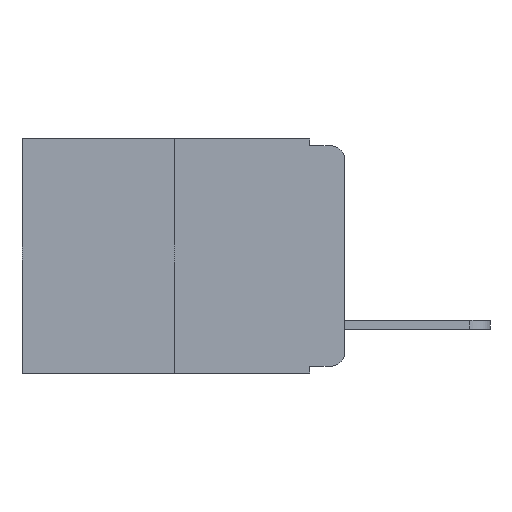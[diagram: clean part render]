
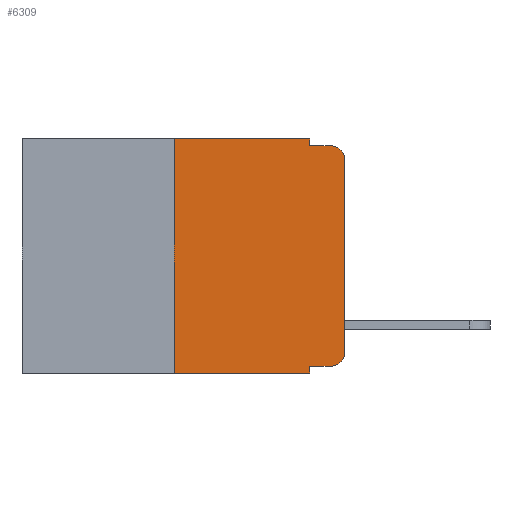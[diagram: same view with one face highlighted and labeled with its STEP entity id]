
A CAD part, left-side view. The second image highlights one B-rep face of the part: STEP entity #6309.
In plain terms, the highlighted planar face has unit normal (-1, 0, 0).
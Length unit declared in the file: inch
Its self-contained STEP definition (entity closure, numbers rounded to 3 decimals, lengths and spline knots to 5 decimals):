
#97 = EDGE_CURVE ( 'NONE', #1226, #12075, #10410, .T. ) ;
#173 = CARTESIAN_POINT ( 'NONE',  ( 0., 0.051, 0. ) ) ;
#277 = EDGE_CURVE ( 'NONE', #12075, #1730, #10878, .T. ) ;
#729 = VERTEX_POINT ( 'NONE', #4508 ) ;
#790 = VECTOR ( 'NONE', #1117, 39.37008 ) ;
#823 = ORIENTED_EDGE ( 'NONE', *, *, #1508, .T. ) ;
#833 = VERTEX_POINT ( 'NONE', #1944 ) ;
#1117 = DIRECTION ( 'NONE',  ( 0., 0., 1. ) ) ;
#1226 = VERTEX_POINT ( 'NONE', #11450 ) ;
#1508 = EDGE_CURVE ( 'NONE', #1730, #5618, #3869, .T. ) ;
#1667 = DIRECTION ( 'NONE',  ( 0., 0., -1. ) ) ;
#1677 = DIRECTION ( 'NONE',  ( -1., 0., 0. ) ) ;
#1699 = CARTESIAN_POINT ( 'NONE',  ( 0., 0.02, -0.313 ) ) ;
#1730 = VERTEX_POINT ( 'NONE', #4477 ) ;
#1927 = ORIENTED_EDGE ( 'NONE', *, *, #9989, .F. ) ;
#1944 = CARTESIAN_POINT ( 'NONE',  ( 0., 0.25, -0.343 ) ) ;
#1975 = VECTOR ( 'NONE', #6902, 39.37008 ) ;
#1986 = CARTESIAN_POINT ( 'NONE',  ( 0., 0., 0. ) ) ;
#2204 = AXIS2_PLACEMENT_3D ( 'NONE', #10571, #10408, #10288 ) ;
#2370 = CARTESIAN_POINT ( 'NONE',  ( 0., 0.25, 0. ) ) ;
#2376 = CARTESIAN_POINT ( 'NONE',  ( 0., 0.02, -0.333 ) ) ;
#2549 = LINE ( 'NONE', #5717, #13097 ) ;
#2639 = VERTEX_POINT ( 'NONE', #9221 ) ;
#2655 = ORIENTED_EDGE ( 'NONE', *, *, #7296, .F. ) ;
#3625 = LINE ( 'NONE', #7556, #9122 ) ;
#3672 = VECTOR ( 'NONE', #12641, 39.37008 ) ;
#3692 = VERTEX_POINT ( 'NONE', #173 ) ;
#3740 = ORIENTED_EDGE ( 'NONE', *, *, #12551, .T. ) ;
#3869 = LINE ( 'NONE', #1986, #790 ) ;
#3941 = CARTESIAN_POINT ( 'NONE',  ( 0., 0., -0.03 ) ) ;
#4017 = VERTEX_POINT ( 'NONE', #8702 ) ;
#4297 = DIRECTION ( 'NONE',  ( 0., 0., 1. ) ) ;
#4322 = CARTESIAN_POINT ( 'NONE',  ( 0., 0.25, 0. ) ) ;
#4477 = CARTESIAN_POINT ( 'NONE',  ( 0., 0., -0.313 ) ) ;
#4508 = CARTESIAN_POINT ( 'NONE',  ( 0., 0.051, -0.01 ) ) ;
#5552 = DIRECTION ( 'NONE',  ( 0., -1., 0. ) ) ;
#5618 = VERTEX_POINT ( 'NONE', #3941 ) ;
#5717 = CARTESIAN_POINT ( 'NONE',  ( 0., 0.473, 0. ) ) ;
#5868 = ORIENTED_EDGE ( 'NONE', *, *, #13182, .F. ) ;
#6282 = CIRCLE ( 'NONE', #12538, 0.02 ) ;
#6309 = ADVANCED_FACE ( 'NONE', ( #7497 ), #10596, .F. ) ;
#6848 = AXIS2_PLACEMENT_3D ( 'NONE', #1699, #1677, #1667 ) ;
#6902 = DIRECTION ( 'NONE',  ( 0., -1., 0. ) ) ;
#6970 = VECTOR ( 'NONE', #8955, 39.37008 ) ;
#6977 = ORIENTED_EDGE ( 'NONE', *, *, #12343, .T. ) ;
#7018 = CARTESIAN_POINT ( 'NONE',  ( 0., 0.051, -0.333 ) ) ;
#7035 = DIRECTION ( 'NONE',  ( 0., 0., -1. ) ) ;
#7059 = CARTESIAN_POINT ( 'NONE',  ( 0., 0.02, -0.03 ) ) ;
#7296 = EDGE_CURVE ( 'NONE', #12074, #3692, #2549, .T. ) ;
#7335 = DIRECTION ( 'NONE',  ( 0., 0., -1. ) ) ;
#7497 = FACE_OUTER_BOUND ( 'NONE', #8108, .T. ) ;
#7514 = LINE ( 'NONE', #13445, #12498 ) ;
#7556 = CARTESIAN_POINT ( 'NONE',  ( 0., 0.051, 0. ) ) ;
#7676 = EDGE_CURVE ( 'NONE', #1226, #4017, #3625, .T. ) ;
#8004 = VECTOR ( 'NONE', #4297, 39.37008 ) ;
#8108 = EDGE_LOOP ( 'NONE', ( #823, #6977, #1927, #10685, #2655, #5868, #3740, #12163, #9900, #13048 ) ) ;
#8702 = CARTESIAN_POINT ( 'NONE',  ( 0., 0.051, -0.343 ) ) ;
#8955 = DIRECTION ( 'NONE',  ( 0., -1., 0. ) ) ;
#9122 = VECTOR ( 'NONE', #7335, 39.37008 ) ;
#9221 = CARTESIAN_POINT ( 'NONE',  ( 0., 0.02, -0.01 ) ) ;
#9343 = CARTESIAN_POINT ( 'NONE',  ( 0., 0.051, -0.01 ) ) ;
#9818 = LINE ( 'NONE', #12719, #3672 ) ;
#9900 = ORIENTED_EDGE ( 'NONE', *, *, #97, .T. ) ;
#9989 = EDGE_CURVE ( 'NONE', #729, #2639, #12302, .T. ) ;
#10288 = DIRECTION ( 'NONE',  ( 0., 0., -1. ) ) ;
#10369 = DIRECTION ( 'NONE',  ( -1., 0., 0. ) ) ;
#10408 = DIRECTION ( 'NONE',  ( 1., 0., 0. ) ) ;
#10410 = LINE ( 'NONE', #7018, #1975 ) ;
#10571 = CARTESIAN_POINT ( 'NONE',  ( 0., 0.473, 0. ) ) ;
#10596 = PLANE ( 'NONE',  #2204 ) ;
#10685 = ORIENTED_EDGE ( 'NONE', *, *, #13420, .F. ) ;
#10721 = LINE ( 'NONE', #4322, #8004 ) ;
#10878 = CIRCLE ( 'NONE', #6848, 0.02 ) ;
#11450 = CARTESIAN_POINT ( 'NONE',  ( 0., 0.051, -0.333 ) ) ;
#11780 = DIRECTION ( 'NONE',  ( 0., 0., -1. ) ) ;
#12074 = VERTEX_POINT ( 'NONE', #2370 ) ;
#12075 = VERTEX_POINT ( 'NONE', #2376 ) ;
#12163 = ORIENTED_EDGE ( 'NONE', *, *, #7676, .F. ) ;
#12302 = LINE ( 'NONE', #9343, #6970 ) ;
#12343 = EDGE_CURVE ( 'NONE', #5618, #2639, #6282, .T. ) ;
#12498 = VECTOR ( 'NONE', #11780, 39.37008 ) ;
#12538 = AXIS2_PLACEMENT_3D ( 'NONE', #7059, #10369, #7035 ) ;
#12551 = EDGE_CURVE ( 'NONE', #833, #4017, #9818, .T. ) ;
#12641 = DIRECTION ( 'NONE',  ( 0., -1., 0. ) ) ;
#12719 = CARTESIAN_POINT ( 'NONE',  ( 0., 0.473, -0.343 ) ) ;
#13048 = ORIENTED_EDGE ( 'NONE', *, *, #277, .T. ) ;
#13097 = VECTOR ( 'NONE', #5552, 39.37008 ) ;
#13182 = EDGE_CURVE ( 'NONE', #833, #12074, #10721, .T. ) ;
#13420 = EDGE_CURVE ( 'NONE', #3692, #729, #7514, .T. ) ;
#13445 = CARTESIAN_POINT ( 'NONE',  ( 0., 0.051, 0. ) ) ;
